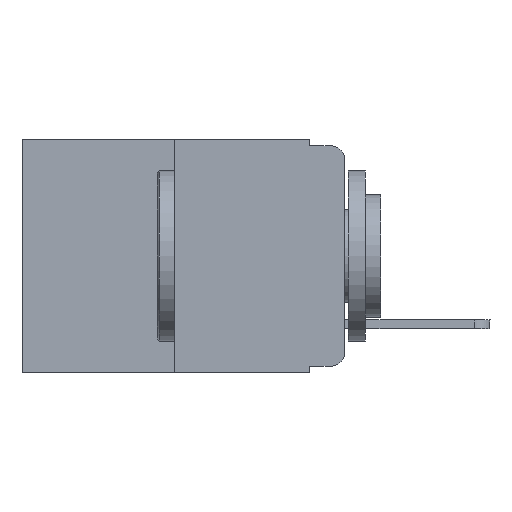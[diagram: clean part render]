
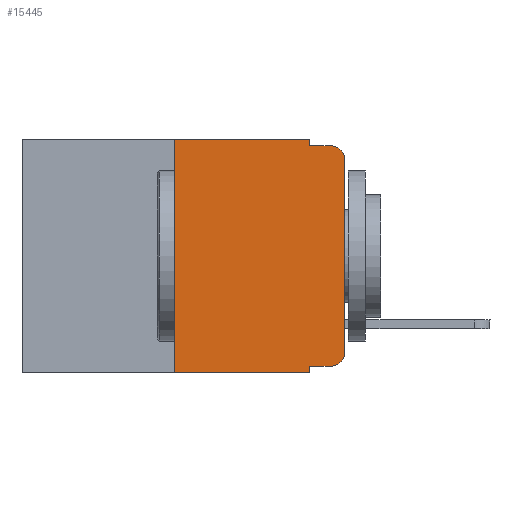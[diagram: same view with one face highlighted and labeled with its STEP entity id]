
A CAD part, left-side view. The second image highlights one B-rep face of the part: STEP entity #15445.
In plain terms, the highlighted planar face has unit normal (-1, 0, 0).
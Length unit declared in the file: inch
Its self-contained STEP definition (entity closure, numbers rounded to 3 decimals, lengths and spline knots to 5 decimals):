
#686 = DIRECTION ( 'NONE',  ( 0., 0., -1. ) ) ;
#886 = EDGE_CURVE ( 'NONE', #2961, #12391, #8853, .T. ) ;
#1118 = EDGE_CURVE ( 'NONE', #23094, #12619, #19107, .T. ) ;
#1285 = VERTEX_POINT ( 'NONE', #3206 ) ;
#1511 = EDGE_CURVE ( 'NONE', #12665, #2961, #21414, .T. ) ;
#2954 = DIRECTION ( 'NONE',  ( 1., 0., 0. ) ) ;
#2961 = VERTEX_POINT ( 'NONE', #3420 ) ;
#3206 = CARTESIAN_POINT ( 'NONE',  ( 0., 0.051, 0. ) ) ;
#3262 = CARTESIAN_POINT ( 'NONE',  ( 0., 0.25, 0. ) ) ;
#3402 = CARTESIAN_POINT ( 'NONE',  ( 0., 0.25, -0.343 ) ) ;
#3420 = CARTESIAN_POINT ( 'NONE',  ( 0., 0.02, -0.333 ) ) ;
#3455 = CARTESIAN_POINT ( 'NONE',  ( 0., 0., -0.03 ) ) ;
#3596 = CIRCLE ( 'NONE', #16289, 0.02 ) ;
#3613 = CARTESIAN_POINT ( 'NONE',  ( 0., 0.473, 0. ) ) ;
#3897 = CARTESIAN_POINT ( 'NONE',  ( 0., 0.051, -0.343 ) ) ;
#4288 = CARTESIAN_POINT ( 'NONE',  ( 0., 0.051, -0.333 ) ) ;
#4609 = CARTESIAN_POINT ( 'NONE',  ( 0., 0.051, -0.333 ) ) ;
#5474 = AXIS2_PLACEMENT_3D ( 'NONE', #21451, #2954, #15945 ) ;
#5747 = LINE ( 'NONE', #19106, #5925 ) ;
#5925 = VECTOR ( 'NONE', #686, 39.37008 ) ;
#6240 = EDGE_CURVE ( 'NONE', #1285, #23094, #12526, .T. ) ;
#6717 = EDGE_CURVE ( 'NONE', #9800, #19288, #23080, .T. ) ;
#7147 = EDGE_CURVE ( 'NONE', #12391, #20087, #12433, .T. ) ;
#7718 = ORIENTED_EDGE ( 'NONE', *, *, #6717, .T. ) ;
#8276 = DIRECTION ( 'NONE',  ( 0., -1., 0. ) ) ;
#8392 = CARTESIAN_POINT ( 'NONE',  ( 0., 0.051, -0.01 ) ) ;
#8816 = ORIENTED_EDGE ( 'NONE', *, *, #17333, .F. ) ;
#8828 = CARTESIAN_POINT ( 'NONE',  ( 0., 0., 0. ) ) ;
#8853 = CIRCLE ( 'NONE', #10015, 0.02 ) ;
#8961 = VECTOR ( 'NONE', #14499, 39.37008 ) ;
#9023 = EDGE_CURVE ( 'NONE', #15212, #1285, #20093, .T. ) ;
#9124 = ORIENTED_EDGE ( 'NONE', *, *, #1511, .T. ) ;
#9275 = VECTOR ( 'NONE', #19858, 39.37008 ) ;
#9497 = CARTESIAN_POINT ( 'NONE',  ( 0., 0.25, 0. ) ) ;
#9800 = VERTEX_POINT ( 'NONE', #3402 ) ;
#10015 = AXIS2_PLACEMENT_3D ( 'NONE', #20966, #10162, #23013 ) ;
#10162 = DIRECTION ( 'NONE',  ( -1., 0., 0. ) ) ;
#10295 = PLANE ( 'NONE',  #5474 ) ;
#10357 = CARTESIAN_POINT ( 'NONE',  ( 0., 0.02, -0.03 ) ) ;
#10376 = DIRECTION ( 'NONE',  ( 0., 0., 1. ) ) ;
#10912 = ORIENTED_EDGE ( 'NONE', *, *, #6240, .F. ) ;
#11077 = DIRECTION ( 'NONE',  ( 0., -1., 0. ) ) ;
#12177 = CARTESIAN_POINT ( 'NONE',  ( 0., 0.051, -0.01 ) ) ;
#12391 = VERTEX_POINT ( 'NONE', #14051 ) ;
#12406 = LINE ( 'NONE', #3262, #21904 ) ;
#12433 = LINE ( 'NONE', #8828, #8961 ) ;
#12526 = LINE ( 'NONE', #17939, #9275 ) ;
#12619 = VERTEX_POINT ( 'NONE', #20284 ) ;
#12665 = VERTEX_POINT ( 'NONE', #4288 ) ;
#12824 = ORIENTED_EDGE ( 'NONE', *, *, #16293, .T. ) ;
#13295 = VECTOR ( 'NONE', #11077, 39.37008 ) ;
#13418 = EDGE_CURVE ( 'NONE', #9800, #15212, #12406, .T. ) ;
#13584 = VECTOR ( 'NONE', #17721, 39.37008 ) ;
#14051 = CARTESIAN_POINT ( 'NONE',  ( 0., 0., -0.313 ) ) ;
#14319 = DIRECTION ( 'NONE',  ( 0., -1., 0. ) ) ;
#14499 = DIRECTION ( 'NONE',  ( 0., 0., 1. ) ) ;
#15212 = VERTEX_POINT ( 'NONE', #9497 ) ;
#15395 = FACE_OUTER_BOUND ( 'NONE', #18191, .T. ) ;
#15445 = ADVANCED_FACE ( 'NONE', ( #15395 ), #10295, .F. ) ;
#15887 = ORIENTED_EDGE ( 'NONE', *, *, #886, .T. ) ;
#15945 = DIRECTION ( 'NONE',  ( 0., 0., -1. ) ) ;
#16289 = AXIS2_PLACEMENT_3D ( 'NONE', #10357, #19369, #19034 ) ;
#16293 = EDGE_CURVE ( 'NONE', #20087, #12619, #3596, .T. ) ;
#17198 = VECTOR ( 'NONE', #14319, 39.37008 ) ;
#17333 = EDGE_CURVE ( 'NONE', #12665, #19288, #5747, .T. ) ;
#17381 = ORIENTED_EDGE ( 'NONE', *, *, #1118, .F. ) ;
#17721 = DIRECTION ( 'NONE',  ( 0., -1., 0. ) ) ;
#17939 = CARTESIAN_POINT ( 'NONE',  ( 0., 0.051, 0. ) ) ;
#18119 = ORIENTED_EDGE ( 'NONE', *, *, #9023, .F. ) ;
#18191 = EDGE_LOOP ( 'NONE', ( #23161, #12824, #17381, #10912, #18119, #20819, #7718, #8816, #9124, #15887 ) ) ;
#19034 = DIRECTION ( 'NONE',  ( 0., 0., -1. ) ) ;
#19106 = CARTESIAN_POINT ( 'NONE',  ( 0., 0.051, 0. ) ) ;
#19107 = LINE ( 'NONE', #8392, #20463 ) ;
#19288 = VERTEX_POINT ( 'NONE', #3897 ) ;
#19356 = CARTESIAN_POINT ( 'NONE',  ( 0., 0.473, -0.343 ) ) ;
#19369 = DIRECTION ( 'NONE',  ( -1., 0., 0. ) ) ;
#19858 = DIRECTION ( 'NONE',  ( 0., 0., -1. ) ) ;
#20087 = VERTEX_POINT ( 'NONE', #3455 ) ;
#20093 = LINE ( 'NONE', #3613, #13295 ) ;
#20284 = CARTESIAN_POINT ( 'NONE',  ( 0., 0.02, -0.01 ) ) ;
#20463 = VECTOR ( 'NONE', #8276, 39.37008 ) ;
#20819 = ORIENTED_EDGE ( 'NONE', *, *, #13418, .F. ) ;
#20966 = CARTESIAN_POINT ( 'NONE',  ( 0., 0.02, -0.313 ) ) ;
#21414 = LINE ( 'NONE', #4609, #13584 ) ;
#21451 = CARTESIAN_POINT ( 'NONE',  ( 0., 0.473, 0. ) ) ;
#21904 = VECTOR ( 'NONE', #10376, 39.37008 ) ;
#23013 = DIRECTION ( 'NONE',  ( 0., 0., -1. ) ) ;
#23080 = LINE ( 'NONE', #19356, #17198 ) ;
#23094 = VERTEX_POINT ( 'NONE', #12177 ) ;
#23161 = ORIENTED_EDGE ( 'NONE', *, *, #7147, .T. ) ;
